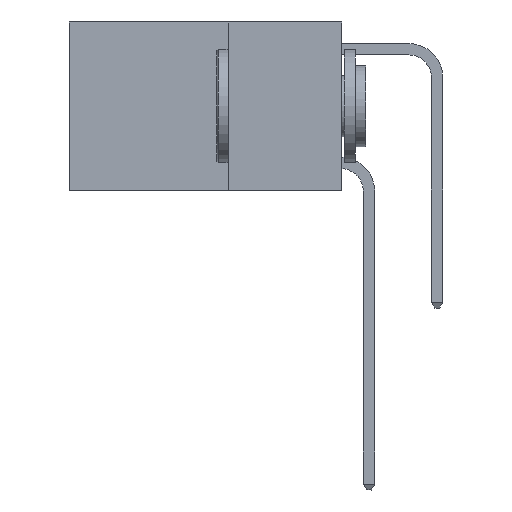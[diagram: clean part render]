
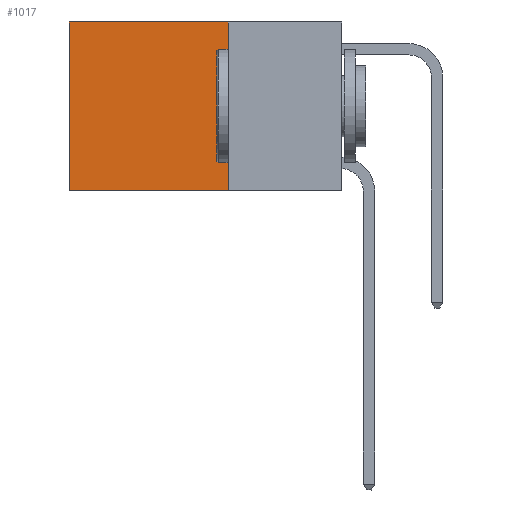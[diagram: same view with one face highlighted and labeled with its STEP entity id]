
A CAD part, left-side view. The second image highlights one B-rep face of the part: STEP entity #1017.
In plain terms, the highlighted planar face has unit normal (-1, 0, 0).
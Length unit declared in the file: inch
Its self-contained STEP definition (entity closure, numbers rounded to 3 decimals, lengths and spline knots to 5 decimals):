
#323 = EDGE_CURVE ( 'NONE', #13836, #14446, #4664, .T. ) ;
#491 = ORIENTED_EDGE ( 'NONE', *, *, #12173, .T. ) ;
#1017 = ADVANCED_FACE ( 'NONE', ( #13166 ), #3799, .F. ) ;
#1872 = LINE ( 'NONE', #3951, #14387 ) ;
#2174 = EDGE_CURVE ( 'NONE', #14669, #13836, #6280, .T. ) ;
#2280 = CARTESIAN_POINT ( 'NONE',  ( 0.2625, 0.25, -0.37 ) ) ;
#2705 = VECTOR ( 'NONE', #15123, 39.37008 ) ;
#3727 = CARTESIAN_POINT ( 'NONE',  ( 0.2625, 0.25, 0. ) ) ;
#3799 = PLANE ( 'NONE',  #5372 ) ;
#3951 = CARTESIAN_POINT ( 'NONE',  ( 0.2625, 0.25, 0. ) ) ;
#4403 = CARTESIAN_POINT ( 'NONE',  ( 0.2625, 0.25, -0.37 ) ) ;
#4573 = VECTOR ( 'NONE', #10241, 39.37008 ) ;
#4664 = LINE ( 'NONE', #2280, #2705 ) ;
#4795 = VECTOR ( 'NONE', #14135, 39.37008 ) ;
#4962 = CARTESIAN_POINT ( 'NONE',  ( 0.2625, 0.6, -0.37 ) ) ;
#5264 = CARTESIAN_POINT ( 'NONE',  ( 0.2625, 0.6, 0. ) ) ;
#5372 = AXIS2_PLACEMENT_3D ( 'NONE', #3727, #8490, #11794 ) ;
#5421 = DIRECTION ( 'NONE',  ( 0., 1., 0. ) ) ;
#6280 = LINE ( 'NONE', #9864, #4573 ) ;
#6544 = EDGE_LOOP ( 'NONE', ( #491, #7712, #13441, #14316 ) ) ;
#6914 = VERTEX_POINT ( 'NONE', #5264 ) ;
#7712 = ORIENTED_EDGE ( 'NONE', *, *, #323, .F. ) ;
#8464 = CARTESIAN_POINT ( 'NONE',  ( 0.2625, 0.6, 0. ) ) ;
#8490 = DIRECTION ( 'NONE',  ( 1., 0., 0. ) ) ;
#9864 = CARTESIAN_POINT ( 'NONE',  ( 0.2625, 0.25, 0. ) ) ;
#10241 = DIRECTION ( 'NONE',  ( 0., 0., -1. ) ) ;
#10662 = EDGE_CURVE ( 'NONE', #14669, #6914, #1872, .T. ) ;
#11428 = CARTESIAN_POINT ( 'NONE',  ( 0.2625, 0.25, 0. ) ) ;
#11794 = DIRECTION ( 'NONE',  ( 0., 0., -1. ) ) ;
#12173 = EDGE_CURVE ( 'NONE', #6914, #14446, #15230, .T. ) ;
#13166 = FACE_OUTER_BOUND ( 'NONE', #6544, .T. ) ;
#13441 = ORIENTED_EDGE ( 'NONE', *, *, #2174, .F. ) ;
#13836 = VERTEX_POINT ( 'NONE', #4403 ) ;
#14135 = DIRECTION ( 'NONE',  ( 0., 0., -1. ) ) ;
#14316 = ORIENTED_EDGE ( 'NONE', *, *, #10662, .T. ) ;
#14387 = VECTOR ( 'NONE', #5421, 39.37008 ) ;
#14446 = VERTEX_POINT ( 'NONE', #4962 ) ;
#14669 = VERTEX_POINT ( 'NONE', #11428 ) ;
#15123 = DIRECTION ( 'NONE',  ( 0., 1., 0. ) ) ;
#15230 = LINE ( 'NONE', #8464, #4795 ) ;
